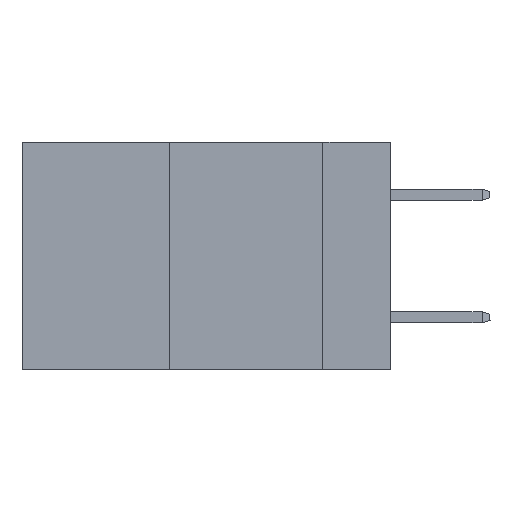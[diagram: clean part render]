
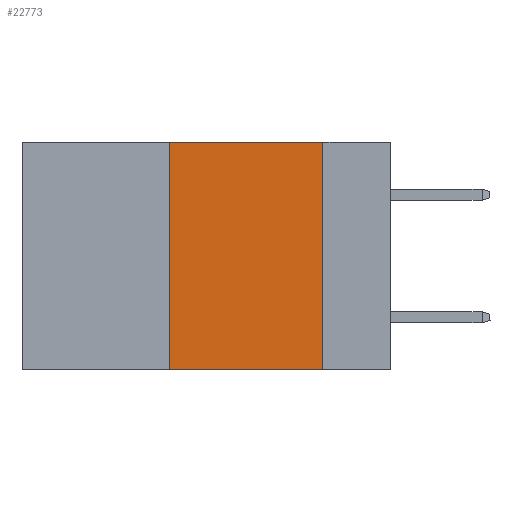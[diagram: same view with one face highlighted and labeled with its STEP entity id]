
A CAD part, left-side view. The second image highlights one B-rep face of the part: STEP entity #22773.
In plain terms, the highlighted planar face has unit normal (-1, 0, 0).
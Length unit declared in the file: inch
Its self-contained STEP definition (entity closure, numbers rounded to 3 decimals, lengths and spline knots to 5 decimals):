
#192 = DIRECTION ( 'NONE',  ( 0., -1., 0. ) ) ;
#1312 = DIRECTION ( 'NONE',  ( 0., 0., -1. ) ) ;
#1935 = VECTOR ( 'NONE', #192, 39.37008 ) ;
#2825 = VERTEX_POINT ( 'NONE', #12780 ) ;
#3136 = CARTESIAN_POINT ( 'NONE',  ( 0., 0.36, 0. ) ) ;
#3568 = ORIENTED_EDGE ( 'NONE', *, *, #13657, .F. ) ;
#4203 = VECTOR ( 'NONE', #6774, 39.37008 ) ;
#4849 = CARTESIAN_POINT ( 'NONE',  ( 0., 0.11, 0. ) ) ;
#6774 = DIRECTION ( 'NONE',  ( 0., 0., 1. ) ) ;
#6901 = ORIENTED_EDGE ( 'NONE', *, *, #10559, .F. ) ;
#7238 = CARTESIAN_POINT ( 'NONE',  ( 0., 0.6, 0. ) ) ;
#7561 = VECTOR ( 'NONE', #12645, 39.37008 ) ;
#8159 = DIRECTION ( 'NONE',  ( 0., 0., -1. ) ) ;
#8255 = DIRECTION ( 'NONE',  ( 1., 0., 0. ) ) ;
#8411 = CARTESIAN_POINT ( 'NONE',  ( 0., 0.6, 0. ) ) ;
#8453 = VERTEX_POINT ( 'NONE', #13814 ) ;
#9111 = LINE ( 'NONE', #20390, #18520 ) ;
#9184 = CARTESIAN_POINT ( 'NONE',  ( 0., 0.6, -0.37 ) ) ;
#9323 = EDGE_CURVE ( 'NONE', #2825, #18069, #16182, .T. ) ;
#10559 = EDGE_CURVE ( 'NONE', #8453, #2825, #19386, .T. ) ;
#10695 = AXIS2_PLACEMENT_3D ( 'NONE', #8411, #8255, #1312 ) ;
#12417 = ORIENTED_EDGE ( 'NONE', *, *, #9323, .F. ) ;
#12645 = DIRECTION ( 'NONE',  ( 0., -1., 0. ) ) ;
#12780 = CARTESIAN_POINT ( 'NONE',  ( 0., 0.36, 0. ) ) ;
#12835 = ORIENTED_EDGE ( 'NONE', *, *, #14030, .T. ) ;
#13657 = EDGE_CURVE ( 'NONE', #18069, #14214, #9111, .T. ) ;
#13814 = CARTESIAN_POINT ( 'NONE',  ( 0., 0.36, -0.37 ) ) ;
#14030 = EDGE_CURVE ( 'NONE', #8453, #14214, #14107, .T. ) ;
#14107 = LINE ( 'NONE', #9184, #1935 ) ;
#14214 = VERTEX_POINT ( 'NONE', #16103 ) ;
#15466 = EDGE_LOOP ( 'NONE', ( #3568, #12417, #6901, #12835 ) ) ;
#16103 = CARTESIAN_POINT ( 'NONE',  ( 0., 0.11, -0.37 ) ) ;
#16182 = LINE ( 'NONE', #7238, #7561 ) ;
#18069 = VERTEX_POINT ( 'NONE', #4849 ) ;
#18520 = VECTOR ( 'NONE', #8159, 39.37008 ) ;
#19386 = LINE ( 'NONE', #3136, #4203 ) ;
#20390 = CARTESIAN_POINT ( 'NONE',  ( 0., 0.11, 0. ) ) ;
#21978 = FACE_OUTER_BOUND ( 'NONE', #15466, .T. ) ;
#22390 = PLANE ( 'NONE',  #10695 ) ;
#22773 = ADVANCED_FACE ( 'NONE', ( #21978 ), #22390, .F. ) ;
